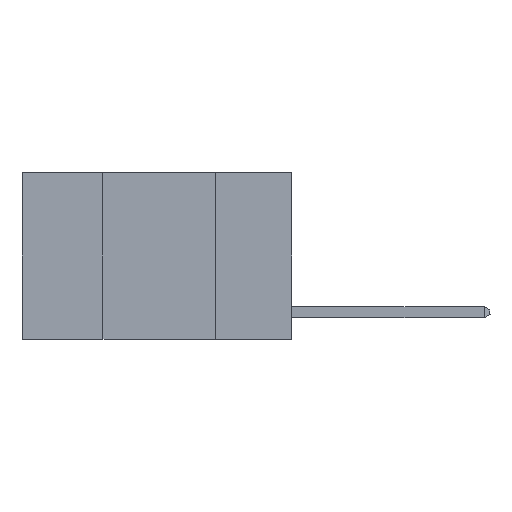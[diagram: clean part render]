
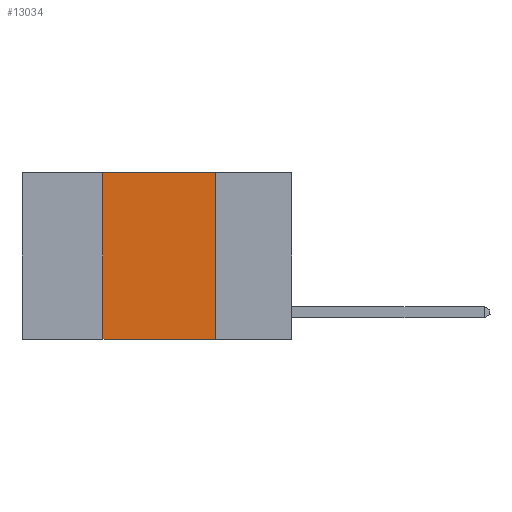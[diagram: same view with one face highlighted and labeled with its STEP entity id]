
A CAD part, left-side view. The second image highlights one B-rep face of the part: STEP entity #13034.
In plain terms, the highlighted planar face has unit normal (-1, 0, 0).
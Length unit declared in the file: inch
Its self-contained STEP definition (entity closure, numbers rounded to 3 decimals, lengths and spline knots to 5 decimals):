
#550 = DIRECTION ( 'NONE',  ( 0., 0., -1. ) ) ;
#715 = CARTESIAN_POINT ( 'NONE',  ( 0., 0.6, 0. ) ) ;
#1756 = EDGE_LOOP ( 'NONE', ( #10933, #9781, #3658, #8269 ) ) ;
#1779 = VERTEX_POINT ( 'NONE', #6284 ) ;
#2052 = FACE_OUTER_BOUND ( 'NONE', #1756, .T. ) ;
#2586 = VECTOR ( 'NONE', #10823, 39.37008 ) ;
#3453 = VERTEX_POINT ( 'NONE', #11267 ) ;
#3658 = ORIENTED_EDGE ( 'NONE', *, *, #12860, .F. ) ;
#3736 = CARTESIAN_POINT ( 'NONE',  ( 0., 0.6, 0. ) ) ;
#3877 = VERTEX_POINT ( 'NONE', #5928 ) ;
#4437 = CARTESIAN_POINT ( 'NONE',  ( 0., 0.17, 0. ) ) ;
#4631 = VECTOR ( 'NONE', #10349, 39.37008 ) ;
#4819 = DIRECTION ( 'NONE',  ( 0., -1., 0. ) ) ;
#5680 = DIRECTION ( 'NONE',  ( 1., 0., 0. ) ) ;
#5928 = CARTESIAN_POINT ( 'NONE',  ( 0., 0.17, -0.37 ) ) ;
#6134 = CARTESIAN_POINT ( 'NONE',  ( 0., 0.6, -0.37 ) ) ;
#6284 = CARTESIAN_POINT ( 'NONE',  ( 0., 0.17, 0. ) ) ;
#6443 = LINE ( 'NONE', #11503, #4631 ) ;
#7457 = VERTEX_POINT ( 'NONE', #13844 ) ;
#7563 = LINE ( 'NONE', #6134, #2586 ) ;
#7852 = VECTOR ( 'NONE', #4819, 39.37008 ) ;
#8197 = DIRECTION ( 'NONE',  ( 0., 0., -1. ) ) ;
#8269 = ORIENTED_EDGE ( 'NONE', *, *, #10832, .T. ) ;
#9523 = PLANE ( 'NONE',  #15564 ) ;
#9781 = ORIENTED_EDGE ( 'NONE', *, *, #13484, .F. ) ;
#9968 = VECTOR ( 'NONE', #8197, 39.37008 ) ;
#10349 = DIRECTION ( 'NONE',  ( 0., 0., 1. ) ) ;
#10823 = DIRECTION ( 'NONE',  ( 0., -1., 0. ) ) ;
#10832 = EDGE_CURVE ( 'NONE', #7457, #3877, #7563, .T. ) ;
#10933 = ORIENTED_EDGE ( 'NONE', *, *, #13015, .F. ) ;
#10968 = LINE ( 'NONE', #3736, #7852 ) ;
#11267 = CARTESIAN_POINT ( 'NONE',  ( 0., 0.42, 0. ) ) ;
#11503 = CARTESIAN_POINT ( 'NONE',  ( 0., 0.42, 0. ) ) ;
#12860 = EDGE_CURVE ( 'NONE', #7457, #3453, #6443, .T. ) ;
#13015 = EDGE_CURVE ( 'NONE', #1779, #3877, #14779, .T. ) ;
#13034 = ADVANCED_FACE ( 'NONE', ( #2052 ), #9523, .F. ) ;
#13484 = EDGE_CURVE ( 'NONE', #3453, #1779, #10968, .T. ) ;
#13844 = CARTESIAN_POINT ( 'NONE',  ( 0., 0.42, -0.37 ) ) ;
#14779 = LINE ( 'NONE', #4437, #9968 ) ;
#15564 = AXIS2_PLACEMENT_3D ( 'NONE', #715, #5680, #550 ) ;
